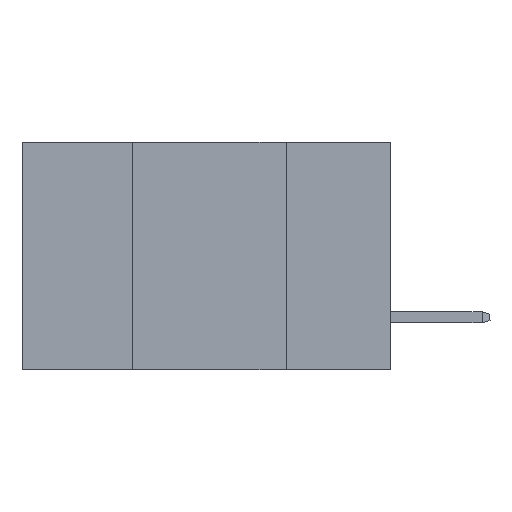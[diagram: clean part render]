
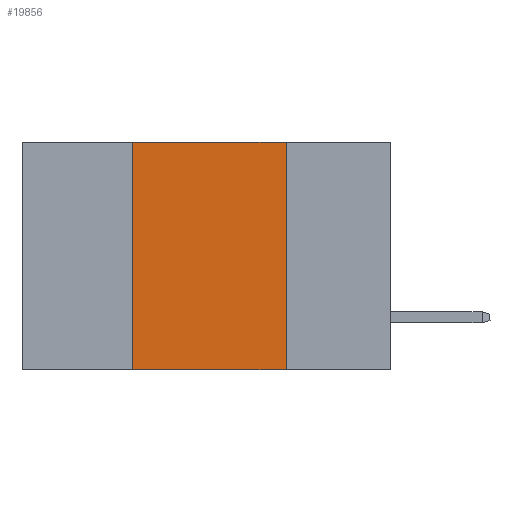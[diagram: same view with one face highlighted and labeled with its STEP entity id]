
A CAD part, left-side view. The second image highlights one B-rep face of the part: STEP entity #19856.
In plain terms, the highlighted planar face has unit normal (-1, 0, 0).
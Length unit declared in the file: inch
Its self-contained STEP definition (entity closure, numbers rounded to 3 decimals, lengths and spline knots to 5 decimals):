
#727 = ORIENTED_EDGE ( 'NONE', *, *, #17118, .F. ) ;
#777 = VERTEX_POINT ( 'NONE', #18312 ) ;
#987 = DIRECTION ( 'NONE',  ( 1., 0., 0. ) ) ;
#1866 = VERTEX_POINT ( 'NONE', #14010 ) ;
#1867 = VERTEX_POINT ( 'NONE', #13800 ) ;
#2282 = VERTEX_POINT ( 'NONE', #9138 ) ;
#2676 = LINE ( 'NONE', #4814, #6809 ) ;
#3029 = DIRECTION ( 'NONE',  ( 0., -1., 0. ) ) ;
#3319 = FACE_OUTER_BOUND ( 'NONE', #12337, .T. ) ;
#4698 = CARTESIAN_POINT ( 'NONE',  ( 0., 0.6, -0.37 ) ) ;
#4814 = CARTESIAN_POINT ( 'NONE',  ( 0., 0.42, 0. ) ) ;
#5300 = CARTESIAN_POINT ( 'NONE',  ( 0., 0.17, 0. ) ) ;
#6131 = EDGE_CURVE ( 'NONE', #2282, #1867, #8560, .T. ) ;
#6359 = DIRECTION ( 'NONE',  ( 0., 0., 1. ) ) ;
#6809 = VECTOR ( 'NONE', #6359, 39.37008 ) ;
#7752 = EDGE_CURVE ( 'NONE', #777, #1867, #8955, .T. ) ;
#8560 = LINE ( 'NONE', #5300, #16280 ) ;
#8563 = DIRECTION ( 'NONE',  ( 0., -1., 0. ) ) ;
#8955 = LINE ( 'NONE', #4698, #16675 ) ;
#9138 = CARTESIAN_POINT ( 'NONE',  ( 0., 0.17, 0. ) ) ;
#10336 = PLANE ( 'NONE',  #15409 ) ;
#11347 = DIRECTION ( 'NONE',  ( 0., 0., -1. ) ) ;
#11886 = DIRECTION ( 'NONE',  ( 0., 0., -1. ) ) ;
#12337 = EDGE_LOOP ( 'NONE', ( #12687, #727, #17705, #14148 ) ) ;
#12687 = ORIENTED_EDGE ( 'NONE', *, *, #6131, .F. ) ;
#13800 = CARTESIAN_POINT ( 'NONE',  ( 0., 0.17, -0.37 ) ) ;
#14010 = CARTESIAN_POINT ( 'NONE',  ( 0., 0.42, 0. ) ) ;
#14148 = ORIENTED_EDGE ( 'NONE', *, *, #7752, .T. ) ;
#14998 = EDGE_CURVE ( 'NONE', #777, #1866, #2676, .T. ) ;
#15188 = LINE ( 'NONE', #17728, #15670 ) ;
#15409 = AXIS2_PLACEMENT_3D ( 'NONE', #19462, #987, #11886 ) ;
#15670 = VECTOR ( 'NONE', #8563, 39.37008 ) ;
#16280 = VECTOR ( 'NONE', #11347, 39.37008 ) ;
#16675 = VECTOR ( 'NONE', #3029, 39.37008 ) ;
#17118 = EDGE_CURVE ( 'NONE', #1866, #2282, #15188, .T. ) ;
#17705 = ORIENTED_EDGE ( 'NONE', *, *, #14998, .F. ) ;
#17728 = CARTESIAN_POINT ( 'NONE',  ( 0., 0.6, 0. ) ) ;
#18312 = CARTESIAN_POINT ( 'NONE',  ( 0., 0.42, -0.37 ) ) ;
#19462 = CARTESIAN_POINT ( 'NONE',  ( 0., 0.6, 0. ) ) ;
#19856 = ADVANCED_FACE ( 'NONE', ( #3319 ), #10336, .F. ) ;
